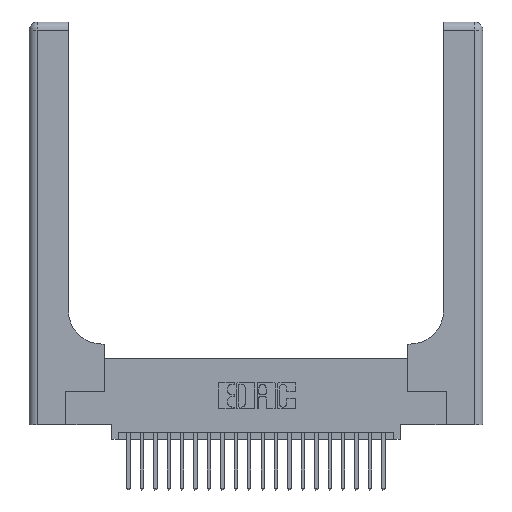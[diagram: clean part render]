
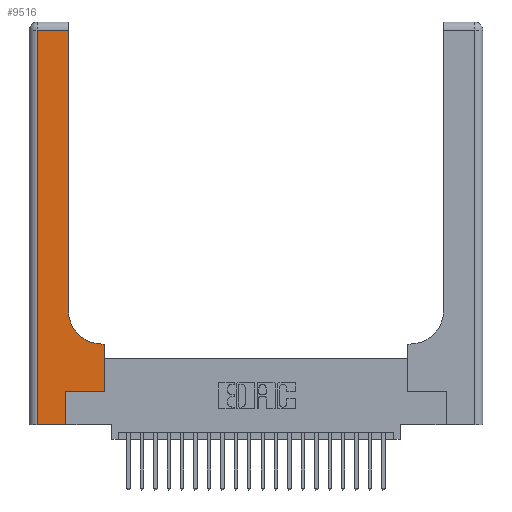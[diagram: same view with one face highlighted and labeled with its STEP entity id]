
A CAD part, top view. The second image highlights one B-rep face of the part: STEP entity #9516.
In plain terms, the highlighted planar face has unit normal (0, 0, 1).
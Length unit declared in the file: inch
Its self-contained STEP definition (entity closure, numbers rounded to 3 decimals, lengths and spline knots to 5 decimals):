
#750 = LINE ( 'NONE', #15065, #9461 ) ;
#771 = CIRCLE ( 'NONE', #14701, 0.25 ) ;
#818 = LINE ( 'NONE', #8631, #4034 ) ;
#1524 = CARTESIAN_POINT ( 'NONE',  ( 0., 3., 0.37 ) ) ;
#2180 = ORIENTED_EDGE ( 'NONE', *, *, #11456, .T. ) ;
#2263 = EDGE_CURVE ( 'NONE', #20363, #8558, #818, .T. ) ;
#2893 = CARTESIAN_POINT ( 'NONE',  ( 0.269, 0.25, 0.37 ) ) ;
#2973 = VECTOR ( 'NONE', #5320, 39.37008 ) ;
#2987 = DIRECTION ( 'NONE',  ( 1., 0., 0. ) ) ;
#3222 = DIRECTION ( 'NONE',  ( 1., 0., 0. ) ) ;
#3250 = CARTESIAN_POINT ( 'NONE',  ( 0.06, 2.94, 0.37 ) ) ;
#3980 = EDGE_CURVE ( 'NONE', #21055, #17015, #750, .T. ) ;
#3991 = DIRECTION ( 'NONE',  ( 0., 1., 0. ) ) ;
#4034 = VECTOR ( 'NONE', #8812, 39.37008 ) ;
#4246 = CARTESIAN_POINT ( 'NONE',  ( 0.2915, 0.6, 0.37 ) ) ;
#4671 = ORIENTED_EDGE ( 'NONE', *, *, #15963, .T. ) ;
#5218 = DIRECTION ( 'NONE',  ( 0., 0., -1. ) ) ;
#5278 = DIRECTION ( 'NONE',  ( 0., 0., -1. ) ) ;
#5320 = DIRECTION ( 'NONE',  ( 0., 1., 0. ) ) ;
#5555 = LINE ( 'NONE', #4246, #9906 ) ;
#6261 = CARTESIAN_POINT ( 'NONE',  ( 0., 0., 0.37 ) ) ;
#6516 = CARTESIAN_POINT ( 'NONE',  ( 0.5415, 0.6, 0.37 ) ) ;
#6720 = VERTEX_POINT ( 'NONE', #6516 ) ;
#7068 = ORIENTED_EDGE ( 'NONE', *, *, #23602, .T. ) ;
#7079 = EDGE_CURVE ( 'NONE', #16384, #7724, #18929, .T. ) ;
#7115 = CARTESIAN_POINT ( 'NONE',  ( 0.06, 3., 0.37 ) ) ;
#7258 = LINE ( 'NONE', #6261, #20344 ) ;
#7724 = VERTEX_POINT ( 'NONE', #23826 ) ;
#7811 = ORIENTED_EDGE ( 'NONE', *, *, #15376, .T. ) ;
#7939 = LINE ( 'NONE', #16604, #10881 ) ;
#8558 = VERTEX_POINT ( 'NONE', #2893 ) ;
#8631 = CARTESIAN_POINT ( 'NONE',  ( 0.269, 0., 0.37 ) ) ;
#8812 = DIRECTION ( 'NONE',  ( 0., 1., 0. ) ) ;
#9060 = DIRECTION ( 'NONE',  ( -1., 0., 0. ) ) ;
#9346 = ORIENTED_EDGE ( 'NONE', *, *, #15331, .T. ) ;
#9461 = VECTOR ( 'NONE', #3991, 39.37008 ) ;
#9516 = ADVANCED_FACE ( 'NONE', ( #22016 ), #23750, .F. ) ;
#9906 = VECTOR ( 'NONE', #9977, 39.37008 ) ;
#9977 = DIRECTION ( 'NONE',  ( -1., 0., 0. ) ) ;
#10265 = CARTESIAN_POINT ( 'NONE',  ( 0.269, 0.25, 0.37 ) ) ;
#10881 = VECTOR ( 'NONE', #20350, 39.37008 ) ;
#11456 = EDGE_CURVE ( 'NONE', #7724, #17340, #7939, .T. ) ;
#11594 = CARTESIAN_POINT ( 'NONE',  ( 0.5585, 0.25, 0.37 ) ) ;
#12203 = ORIENTED_EDGE ( 'NONE', *, *, #14038, .T. ) ;
#12449 = ORIENTED_EDGE ( 'NONE', *, *, #2263, .T. ) ;
#13294 = CARTESIAN_POINT ( 'NONE',  ( 0.2915, 0.85, 0.37 ) ) ;
#13685 = CARTESIAN_POINT ( 'NONE',  ( 0.5585, 0.6, 0.37 ) ) ;
#14038 = EDGE_CURVE ( 'NONE', #17801, #20363, #7258, .T. ) ;
#14701 = AXIS2_PLACEMENT_3D ( 'NONE', #16400, #5278, #18286 ) ;
#14724 = CARTESIAN_POINT ( 'NONE',  ( 0.269, 0., 0.37 ) ) ;
#15065 = CARTESIAN_POINT ( 'NONE',  ( 0.5585, 0.25, 0.37 ) ) ;
#15331 = EDGE_CURVE ( 'NONE', #17340, #17801, #15593, .T. ) ;
#15376 = EDGE_CURVE ( 'NONE', #8558, #21055, #17074, .T. ) ;
#15593 = LINE ( 'NONE', #7115, #22028 ) ;
#15963 = EDGE_CURVE ( 'NONE', #6720, #16384, #771, .T. ) ;
#16384 = VERTEX_POINT ( 'NONE', #13294 ) ;
#16400 = CARTESIAN_POINT ( 'NONE',  ( 0.5415, 0.85, 0.37 ) ) ;
#16604 = CARTESIAN_POINT ( 'NONE',  ( 0., 2.94, 0.37 ) ) ;
#17015 = VERTEX_POINT ( 'NONE', #13685 ) ;
#17074 = LINE ( 'NONE', #10265, #20273 ) ;
#17340 = VERTEX_POINT ( 'NONE', #3250 ) ;
#17412 = ORIENTED_EDGE ( 'NONE', *, *, #3980, .T. ) ;
#17562 = CARTESIAN_POINT ( 'NONE',  ( 0.06, 0., 0.37 ) ) ;
#17801 = VERTEX_POINT ( 'NONE', #17562 ) ;
#18286 = DIRECTION ( 'NONE',  ( 1., 0., 0. ) ) ;
#18913 = ORIENTED_EDGE ( 'NONE', *, *, #7079, .T. ) ;
#18929 = LINE ( 'NONE', #22831, #2973 ) ;
#19895 = AXIS2_PLACEMENT_3D ( 'NONE', #1524, #5218, #9060 ) ;
#20112 = DIRECTION ( 'NONE',  ( 0., -1., 0. ) ) ;
#20273 = VECTOR ( 'NONE', #2987, 39.37008 ) ;
#20344 = VECTOR ( 'NONE', #3222, 39.37008 ) ;
#20350 = DIRECTION ( 'NONE',  ( -1., 0., 0. ) ) ;
#20363 = VERTEX_POINT ( 'NONE', #14724 ) ;
#21055 = VERTEX_POINT ( 'NONE', #11594 ) ;
#22016 = FACE_OUTER_BOUND ( 'NONE', #23452, .T. ) ;
#22028 = VECTOR ( 'NONE', #20112, 39.37008 ) ;
#22831 = CARTESIAN_POINT ( 'NONE',  ( 0.2915, 3., 0.37 ) ) ;
#23452 = EDGE_LOOP ( 'NONE', ( #18913, #2180, #9346, #12203, #12449, #7811, #17412, #7068, #4671 ) ) ;
#23602 = EDGE_CURVE ( 'NONE', #17015, #6720, #5555, .T. ) ;
#23750 = PLANE ( 'NONE',  #19895 ) ;
#23826 = CARTESIAN_POINT ( 'NONE',  ( 0.2915, 2.94, 0.37 ) ) ;
